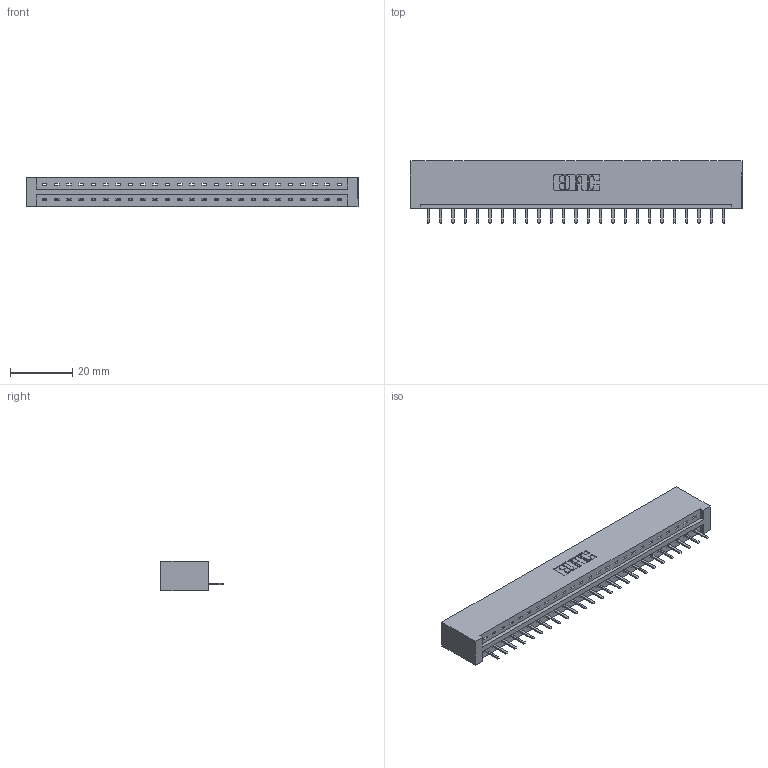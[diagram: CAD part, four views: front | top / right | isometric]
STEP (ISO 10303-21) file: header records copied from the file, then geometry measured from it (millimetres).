
FILE_DESCRIPTION (( 'STEP AP203' ), '1' );
FILE_NAME ('337-025-520-101.STEP', '2018-08-06T02:27:37', ( '' ), ( '' ), 'SwSTEP 2.0', 'SolidWorks 2016', '' );
FILE_SCHEMA (( 'CONFIG_CONTROL_DESIGN' ));
Length unit declared in the file: inch
Products named in the file (3): 337 Part_No Mounting Lugs; 345-292-001_345-293-120; 337-025-520-101
Assembly tree (26 placements, depth 2):
  337-025-520-101
    337 Part_No Mounting Lugs
    345-292-001_345-293-120  x25
Bounding box: 106.93 x 20.02 x 9.4 mm (x, y, z)
Volume: 11568.1 mm3; surface area: 11582.1 mm2
Topology: 26 solids, 26 shells, 1756 faces, 5187 edges, 3390 vertices
Faces by surface type: plane 1266, cylinder 490
Entity records: 20619 total; most frequent: CARTESIAN_POINT 3609, ORIENTED_EDGE 3558, DIRECTION 3053, EDGE_CURVE 1779, VECTOR 1655, LINE 1655, VERTEX_POINT 1182, AXIS2_PLACEMENT_3D 699
